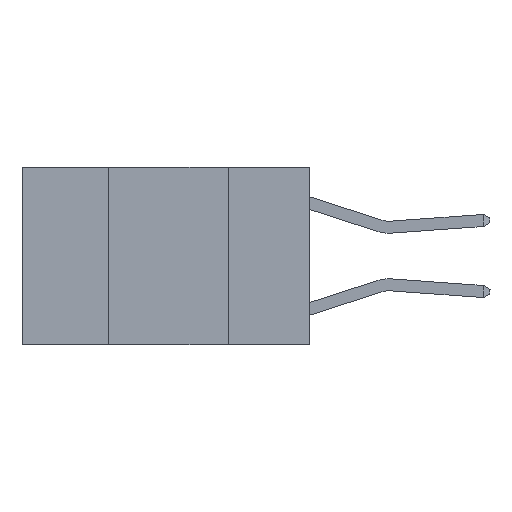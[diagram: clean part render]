
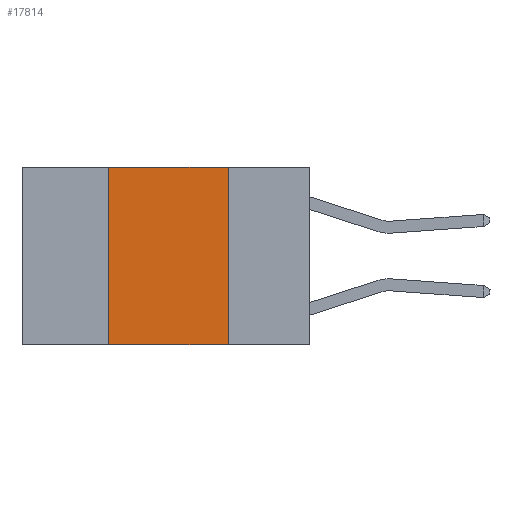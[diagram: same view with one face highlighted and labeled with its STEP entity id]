
A CAD part, left-side view. The second image highlights one B-rep face of the part: STEP entity #17814.
In plain terms, the highlighted planar face has unit normal (-1, 0, 0).
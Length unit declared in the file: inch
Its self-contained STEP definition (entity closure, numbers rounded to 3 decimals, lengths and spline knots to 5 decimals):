
#927 = ORIENTED_EDGE ( 'NONE', *, *, #21329, .T. ) ;
#1484 = FACE_OUTER_BOUND ( 'NONE', #24892, .T. ) ;
#1685 = EDGE_CURVE ( 'NONE', #20725, #16986, #17675, .T. ) ;
#2332 = LINE ( 'NONE', #12501, #12630 ) ;
#2793 = AXIS2_PLACEMENT_3D ( 'NONE', #17695, #4564, #19914 ) ;
#3159 = EDGE_CURVE ( 'NONE', #21498, #12329, #22463, .T. ) ;
#3981 = CARTESIAN_POINT ( 'NONE',  ( 0., 0.42, -0.37 ) ) ;
#4564 = DIRECTION ( 'NONE',  ( 1., 0., 0. ) ) ;
#5364 = ORIENTED_EDGE ( 'NONE', *, *, #3159, .F. ) ;
#5811 = LINE ( 'NONE', #6198, #22601 ) ;
#6198 = CARTESIAN_POINT ( 'NONE',  ( 0., 0.6, 0. ) ) ;
#8836 = DIRECTION ( 'NONE',  ( 0., 0., -1. ) ) ;
#10531 = DIRECTION ( 'NONE',  ( 0., -1., 0. ) ) ;
#10626 = CARTESIAN_POINT ( 'NONE',  ( 0., 0.42, 0. ) ) ;
#11866 = VECTOR ( 'NONE', #19338, 39.37008 ) ;
#12329 = VERTEX_POINT ( 'NONE', #14898 ) ;
#12482 = CARTESIAN_POINT ( 'NONE',  ( 0., 0.42, 0. ) ) ;
#12501 = CARTESIAN_POINT ( 'NONE',  ( 0., 0.6, -0.37 ) ) ;
#12630 = VECTOR ( 'NONE', #25603, 39.37008 ) ;
#12961 = CARTESIAN_POINT ( 'NONE',  ( 0., 0.17, 0. ) ) ;
#13691 = EDGE_CURVE ( 'NONE', #16986, #21498, #5811, .T. ) ;
#14898 = CARTESIAN_POINT ( 'NONE',  ( 0., 0.17, -0.37 ) ) ;
#15497 = PLANE ( 'NONE',  #2793 ) ;
#16986 = VERTEX_POINT ( 'NONE', #12482 ) ;
#17015 = ORIENTED_EDGE ( 'NONE', *, *, #13691, .F. ) ;
#17538 = CARTESIAN_POINT ( 'NONE',  ( 0., 0.17, 0. ) ) ;
#17675 = LINE ( 'NONE', #10626, #11866 ) ;
#17695 = CARTESIAN_POINT ( 'NONE',  ( 0., 0.6, 0. ) ) ;
#17814 = ADVANCED_FACE ( 'NONE', ( #1484 ), #15497, .F. ) ;
#19338 = DIRECTION ( 'NONE',  ( 0., 0., 1. ) ) ;
#19914 = DIRECTION ( 'NONE',  ( 0., 0., -1. ) ) ;
#20725 = VERTEX_POINT ( 'NONE', #3981 ) ;
#21329 = EDGE_CURVE ( 'NONE', #20725, #12329, #2332, .T. ) ;
#21498 = VERTEX_POINT ( 'NONE', #12961 ) ;
#22463 = LINE ( 'NONE', #17538, #23833 ) ;
#22601 = VECTOR ( 'NONE', #10531, 39.37008 ) ;
#22856 = ORIENTED_EDGE ( 'NONE', *, *, #1685, .F. ) ;
#23833 = VECTOR ( 'NONE', #8836, 39.37008 ) ;
#24892 = EDGE_LOOP ( 'NONE', ( #5364, #17015, #22856, #927 ) ) ;
#25603 = DIRECTION ( 'NONE',  ( 0., -1., 0. ) ) ;
